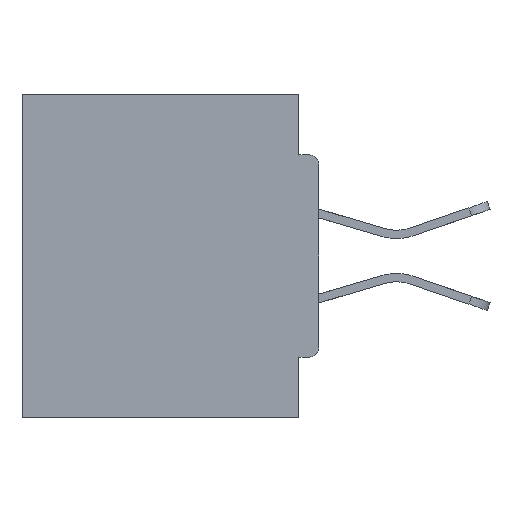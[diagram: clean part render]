
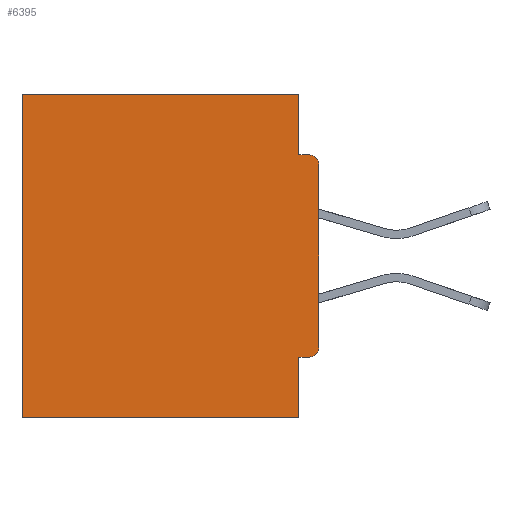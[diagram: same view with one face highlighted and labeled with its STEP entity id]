
A CAD part, left-side view. The second image highlights one B-rep face of the part: STEP entity #6395.
In plain terms, the highlighted planar face has unit normal (-1, 0, 0).
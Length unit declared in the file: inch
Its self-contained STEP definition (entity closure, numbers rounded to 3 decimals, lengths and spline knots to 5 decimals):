
#316 = AXIS2_PLACEMENT_3D ( 'NONE', #7995, #32770, #15930 ) ;
#427 = ORIENTED_EDGE ( 'NONE', *, *, #3442, .F. ) ;
#767 = CARTESIAN_POINT ( 'NONE',  ( 0.298, 0.031, -0.4065 ) ) ;
#1104 = DIRECTION ( 'NONE',  ( 0., 0., -1. ) ) ;
#1296 = CARTESIAN_POINT ( 'NONE',  ( 0.298, 0.015, -0.3915 ) ) ;
#2239 = CARTESIAN_POINT ( 'NONE',  ( 0.298, 0.031, -0.5 ) ) ;
#2644 = CARTESIAN_POINT ( 'NONE',  ( 0.298, 0., -0.4065 ) ) ;
#2944 = LINE ( 'NONE', #6819, #27604 ) ;
#3442 = EDGE_CURVE ( 'NONE', #22277, #17645, #13349, .T. ) ;
#3669 = PLANE ( 'NONE',  #3737 ) ;
#3737 = AXIS2_PLACEMENT_3D ( 'NONE', #14592, #20039, #33988 ) ;
#3772 = ORIENTED_EDGE ( 'NONE', *, *, #34713, .T. ) ;
#3978 = CARTESIAN_POINT ( 'NONE',  ( 0.298, 0., 0. ) ) ;
#4493 = DIRECTION ( 'NONE',  ( 0., 0., -1. ) ) ;
#4823 = EDGE_CURVE ( 'NONE', #9431, #15209, #31227, .T. ) ;
#4862 = ORIENTED_EDGE ( 'NONE', *, *, #9313, .F. ) ;
#5813 = LINE ( 'NONE', #9735, #18544 ) ;
#6395 = ADVANCED_FACE ( 'NONE', ( #22562 ), #3669, .F. ) ;
#6476 = DIRECTION ( 'NONE',  ( -1., 0., 0. ) ) ;
#6819 = CARTESIAN_POINT ( 'NONE',  ( 0.298, 0., -0.0935 ) ) ;
#7540 = LINE ( 'NONE', #33792, #31384 ) ;
#7995 = CARTESIAN_POINT ( 'NONE',  ( 0.298, 0.015, -0.1085 ) ) ;
#8504 = LINE ( 'NONE', #2644, #21219 ) ;
#8842 = CARTESIAN_POINT ( 'NONE',  ( 0.298, 0., -0.3915 ) ) ;
#9313 = EDGE_CURVE ( 'NONE', #15209, #23876, #2944, .T. ) ;
#9431 = VERTEX_POINT ( 'NONE', #35187 ) ;
#9735 = CARTESIAN_POINT ( 'NONE',  ( 0.298, 0.46, 0. ) ) ;
#9757 = CARTESIAN_POINT ( 'NONE',  ( 0.298, 0.031, -0.5 ) ) ;
#10117 = EDGE_CURVE ( 'NONE', #19211, #27470, #35182, .T. ) ;
#10270 = DIRECTION ( 'NONE',  ( 0., 0., -1. ) ) ;
#11582 = VERTEX_POINT ( 'NONE', #29485 ) ;
#13349 = LINE ( 'NONE', #17053, #30428 ) ;
#14053 = CARTESIAN_POINT ( 'NONE',  ( 0.298, 0.015, -0.0935 ) ) ;
#14539 = EDGE_CURVE ( 'NONE', #21684, #22277, #27844, .T. ) ;
#14592 = CARTESIAN_POINT ( 'NONE',  ( 0.298, 0., 0. ) ) ;
#15209 = VERTEX_POINT ( 'NONE', #26389 ) ;
#15251 = CARTESIAN_POINT ( 'NONE',  ( 0.298, 0.031, -0.5 ) ) ;
#15930 = DIRECTION ( 'NONE',  ( 0., 0., -1. ) ) ;
#16706 = VECTOR ( 'NONE', #10270, 39.37008 ) ;
#17053 = CARTESIAN_POINT ( 'NONE',  ( 0.298, 0., -0.5 ) ) ;
#17431 = ORIENTED_EDGE ( 'NONE', *, *, #14539, .F. ) ;
#17645 = VERTEX_POINT ( 'NONE', #24903 ) ;
#17752 = CIRCLE ( 'NONE', #30038, 0.015 ) ;
#18006 = EDGE_CURVE ( 'NONE', #20851, #21684, #8504, .T. ) ;
#18544 = VECTOR ( 'NONE', #4493, 39.37008 ) ;
#18840 = ORIENTED_EDGE ( 'NONE', *, *, #19240, .T. ) ;
#19211 = VERTEX_POINT ( 'NONE', #19963 ) ;
#19240 = EDGE_CURVE ( 'NONE', #9431, #11582, #7540, .T. ) ;
#19413 = VECTOR ( 'NONE', #1104, 39.37008 ) ;
#19963 = CARTESIAN_POINT ( 'NONE',  ( 0.298, 0., -0.1085 ) ) ;
#19999 = CARTESIAN_POINT ( 'NONE',  ( 0.298, 0.015, -0.4065 ) ) ;
#20039 = DIRECTION ( 'NONE',  ( 1., 0., 0. ) ) ;
#20851 = VERTEX_POINT ( 'NONE', #19999 ) ;
#21219 = VECTOR ( 'NONE', #32541, 39.37008 ) ;
#21589 = ORIENTED_EDGE ( 'NONE', *, *, #10117, .F. ) ;
#21684 = VERTEX_POINT ( 'NONE', #767 ) ;
#22277 = VERTEX_POINT ( 'NONE', #2239 ) ;
#22562 = FACE_OUTER_BOUND ( 'NONE', #24342, .T. ) ;
#23876 = VERTEX_POINT ( 'NONE', #14053 ) ;
#24337 = ORIENTED_EDGE ( 'NONE', *, *, #18006, .F. ) ;
#24342 = EDGE_LOOP ( 'NONE', ( #32533, #4862, #26322, #18840, #30633, #427, #17431, #24337, #3772, #21589 ) ) ;
#24903 = CARTESIAN_POINT ( 'NONE',  ( 0.298, 0.46, -0.5 ) ) ;
#25566 = DIRECTION ( 'NONE',  ( 0., 0., -1. ) ) ;
#25692 = DIRECTION ( 'NONE',  ( 0., 1., 0. ) ) ;
#26322 = ORIENTED_EDGE ( 'NONE', *, *, #4823, .F. ) ;
#26389 = CARTESIAN_POINT ( 'NONE',  ( 0.298, 0.031, -0.0935 ) ) ;
#26622 = EDGE_CURVE ( 'NONE', #11582, #17645, #5813, .T. ) ;
#27185 = DIRECTION ( 'NONE',  ( 0., 0., -1. ) ) ;
#27470 = VERTEX_POINT ( 'NONE', #8842 ) ;
#27604 = VECTOR ( 'NONE', #31307, 39.37008 ) ;
#27844 = LINE ( 'NONE', #9757, #32125 ) ;
#28374 = DIRECTION ( 'NONE',  ( 0., 1., 0. ) ) ;
#29485 = CARTESIAN_POINT ( 'NONE',  ( 0.298, 0.46, 0. ) ) ;
#29598 = EDGE_CURVE ( 'NONE', #19211, #23876, #30304, .T. ) ;
#30038 = AXIS2_PLACEMENT_3D ( 'NONE', #1296, #6476, #27185 ) ;
#30304 = CIRCLE ( 'NONE', #316, 0.015 ) ;
#30428 = VECTOR ( 'NONE', #28374, 39.37008 ) ;
#30633 = ORIENTED_EDGE ( 'NONE', *, *, #26622, .T. ) ;
#31227 = LINE ( 'NONE', #15251, #16706 ) ;
#31307 = DIRECTION ( 'NONE',  ( 0., -1., 0. ) ) ;
#31384 = VECTOR ( 'NONE', #25692, 39.37008 ) ;
#32125 = VECTOR ( 'NONE', #25566, 39.37008 ) ;
#32533 = ORIENTED_EDGE ( 'NONE', *, *, #29598, .T. ) ;
#32541 = DIRECTION ( 'NONE',  ( 0., 1., 0. ) ) ;
#32770 = DIRECTION ( 'NONE',  ( -1., 0., 0. ) ) ;
#33792 = CARTESIAN_POINT ( 'NONE',  ( 0.298, 0., 0. ) ) ;
#33988 = DIRECTION ( 'NONE',  ( 0., 0., -1. ) ) ;
#34713 = EDGE_CURVE ( 'NONE', #20851, #27470, #17752, .T. ) ;
#35182 = LINE ( 'NONE', #3978, #19413 ) ;
#35187 = CARTESIAN_POINT ( 'NONE',  ( 0.298, 0.031, 0. ) ) ;
